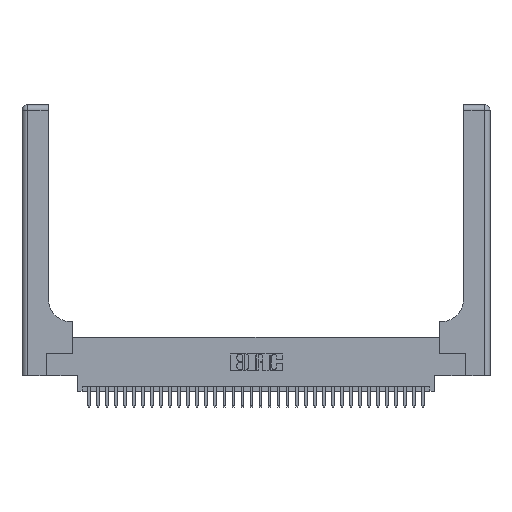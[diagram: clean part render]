
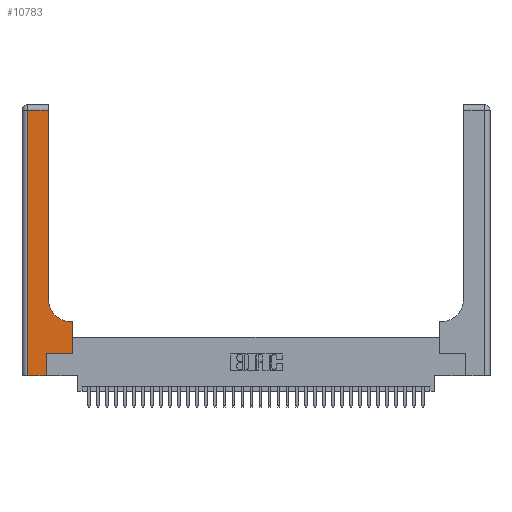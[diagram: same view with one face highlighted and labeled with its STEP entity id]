
A CAD part, top view. The second image highlights one B-rep face of the part: STEP entity #10783.
In plain terms, the highlighted planar face has unit normal (0, 0, 1).
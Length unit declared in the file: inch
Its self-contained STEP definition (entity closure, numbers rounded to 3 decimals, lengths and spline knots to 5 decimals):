
#270 = VERTEX_POINT ( 'NONE', #31087 ) ;
#1474 = VECTOR ( 'NONE', #23679, 39.37008 ) ;
#1972 = AXIS2_PLACEMENT_3D ( 'NONE', #24116, #33994, #29089 ) ;
#2711 = VERTEX_POINT ( 'NONE', #6977 ) ;
#2798 = VERTEX_POINT ( 'NONE', #4079 ) ;
#3326 = CARTESIAN_POINT ( 'NONE',  ( 0., 3., 0.37 ) ) ;
#3829 = CARTESIAN_POINT ( 'NONE',  ( 0.06, 3., 0.37 ) ) ;
#4079 = CARTESIAN_POINT ( 'NONE',  ( 0.2915, 2.94, 0.37 ) ) ;
#4202 = FACE_OUTER_BOUND ( 'NONE', #9363, .T. ) ;
#4945 = VERTEX_POINT ( 'NONE', #11863 ) ;
#6075 = VERTEX_POINT ( 'NONE', #15567 ) ;
#6362 = EDGE_CURVE ( 'NONE', #6075, #2711, #16295, .T. ) ;
#6790 = CARTESIAN_POINT ( 'NONE',  ( 0.2915, 3., 0.37 ) ) ;
#6977 = CARTESIAN_POINT ( 'NONE',  ( 0.06, 0., 0.37 ) ) ;
#7347 = EDGE_CURVE ( 'NONE', #9889, #2798, #23076, .T. ) ;
#7782 = EDGE_CURVE ( 'NONE', #2798, #6075, #17465, .T. ) ;
#8069 = ORIENTED_EDGE ( 'NONE', *, *, #34009, .T. ) ;
#8186 = VECTOR ( 'NONE', #35663, 39.37008 ) ;
#8921 = PLANE ( 'NONE',  #30168 ) ;
#9363 = EDGE_LOOP ( 'NONE', ( #15030, #32447, #27951, #9523, #8069, #18546, #14250, #12564, #28008 ) ) ;
#9523 = ORIENTED_EDGE ( 'NONE', *, *, #30942, .T. ) ;
#9889 = VERTEX_POINT ( 'NONE', #28190 ) ;
#10006 = EDGE_CURVE ( 'NONE', #4945, #27972, #27115, .T. ) ;
#10139 = CARTESIAN_POINT ( 'NONE',  ( 0.269, 0., 0.37 ) ) ;
#10228 = CARTESIAN_POINT ( 'NONE',  ( 0.269, 0.25, 0.37 ) ) ;
#10783 = ADVANCED_FACE ( 'NONE', ( #4202 ), #8921, .F. ) ;
#11863 = CARTESIAN_POINT ( 'NONE',  ( 0.269, 0.25, 0.37 ) ) ;
#12564 = ORIENTED_EDGE ( 'NONE', *, *, #28349, .T. ) ;
#13553 = CIRCLE ( 'NONE', #1972, 0.25 ) ;
#14250 = ORIENTED_EDGE ( 'NONE', *, *, #17570, .T. ) ;
#14374 = DIRECTION ( 'NONE',  ( -1., 0., 0. ) ) ;
#15030 = ORIENTED_EDGE ( 'NONE', *, *, #7347, .T. ) ;
#15264 = VERTEX_POINT ( 'NONE', #30253 ) ;
#15544 = LINE ( 'NONE', #33379, #8186 ) ;
#15567 = CARTESIAN_POINT ( 'NONE',  ( 0.06, 2.94, 0.37 ) ) ;
#16286 = DIRECTION ( 'NONE',  ( 0., 1., 0. ) ) ;
#16295 = LINE ( 'NONE', #3829, #34420 ) ;
#17242 = DIRECTION ( 'NONE',  ( 0., 0., -1. ) ) ;
#17465 = LINE ( 'NONE', #24232, #20910 ) ;
#17570 = EDGE_CURVE ( 'NONE', #27972, #15264, #27031, .T. ) ;
#18546 = ORIENTED_EDGE ( 'NONE', *, *, #10006, .T. ) ;
#19065 = CARTESIAN_POINT ( 'NONE',  ( 0.5585, 0.25, 0.37 ) ) ;
#20096 = LINE ( 'NONE', #32823, #26527 ) ;
#20290 = EDGE_CURVE ( 'NONE', #22905, #9889, #13553, .T. ) ;
#20910 = VECTOR ( 'NONE', #32706, 39.37008 ) ;
#21779 = CARTESIAN_POINT ( 'NONE',  ( 0.5415, 0.6, 0.37 ) ) ;
#22905 = VERTEX_POINT ( 'NONE', #21779 ) ;
#23076 = LINE ( 'NONE', #6790, #1474 ) ;
#23679 = DIRECTION ( 'NONE',  ( 0., 1., 0. ) ) ;
#24116 = CARTESIAN_POINT ( 'NONE',  ( 0.5415, 0.85, 0.37 ) ) ;
#24232 = CARTESIAN_POINT ( 'NONE',  ( 0., 2.94, 0.37 ) ) ;
#25906 = LINE ( 'NONE', #10139, #29369 ) ;
#26258 = VECTOR ( 'NONE', #29704, 39.37008 ) ;
#26527 = VECTOR ( 'NONE', #30228, 39.37008 ) ;
#27031 = LINE ( 'NONE', #30890, #31762 ) ;
#27115 = LINE ( 'NONE', #10228, #26258 ) ;
#27951 = ORIENTED_EDGE ( 'NONE', *, *, #6362, .T. ) ;
#27972 = VERTEX_POINT ( 'NONE', #19065 ) ;
#28008 = ORIENTED_EDGE ( 'NONE', *, *, #20290, .T. ) ;
#28190 = CARTESIAN_POINT ( 'NONE',  ( 0.2915, 0.85, 0.37 ) ) ;
#28349 = EDGE_CURVE ( 'NONE', #15264, #22905, #15544, .T. ) ;
#29089 = DIRECTION ( 'NONE',  ( 1., 0., 0. ) ) ;
#29369 = VECTOR ( 'NONE', #16286, 39.37008 ) ;
#29704 = DIRECTION ( 'NONE',  ( 1., 0., 0. ) ) ;
#30168 = AXIS2_PLACEMENT_3D ( 'NONE', #3326, #17242, #14374 ) ;
#30228 = DIRECTION ( 'NONE',  ( 1., 0., 0. ) ) ;
#30253 = CARTESIAN_POINT ( 'NONE',  ( 0.5585, 0.6, 0.37 ) ) ;
#30645 = DIRECTION ( 'NONE',  ( 0., 1., 0. ) ) ;
#30890 = CARTESIAN_POINT ( 'NONE',  ( 0.5585, 0.25, 0.37 ) ) ;
#30942 = EDGE_CURVE ( 'NONE', #2711, #270, #20096, .T. ) ;
#31087 = CARTESIAN_POINT ( 'NONE',  ( 0.269, 0., 0.37 ) ) ;
#31571 = DIRECTION ( 'NONE',  ( 0., -1., 0. ) ) ;
#31762 = VECTOR ( 'NONE', #30645, 39.37008 ) ;
#32447 = ORIENTED_EDGE ( 'NONE', *, *, #7782, .T. ) ;
#32706 = DIRECTION ( 'NONE',  ( -1., 0., 0. ) ) ;
#32823 = CARTESIAN_POINT ( 'NONE',  ( 0., 0., 0.37 ) ) ;
#33379 = CARTESIAN_POINT ( 'NONE',  ( 0.2915, 0.6, 0.37 ) ) ;
#33994 = DIRECTION ( 'NONE',  ( 0., 0., -1. ) ) ;
#34009 = EDGE_CURVE ( 'NONE', #270, #4945, #25906, .T. ) ;
#34420 = VECTOR ( 'NONE', #31571, 39.37008 ) ;
#35663 = DIRECTION ( 'NONE',  ( -1., 0., 0. ) ) ;
